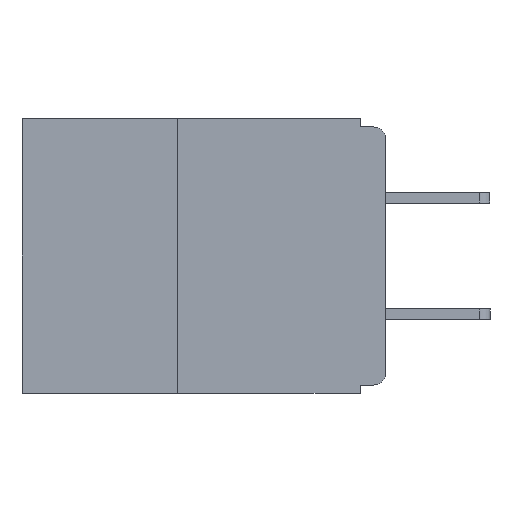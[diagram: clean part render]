
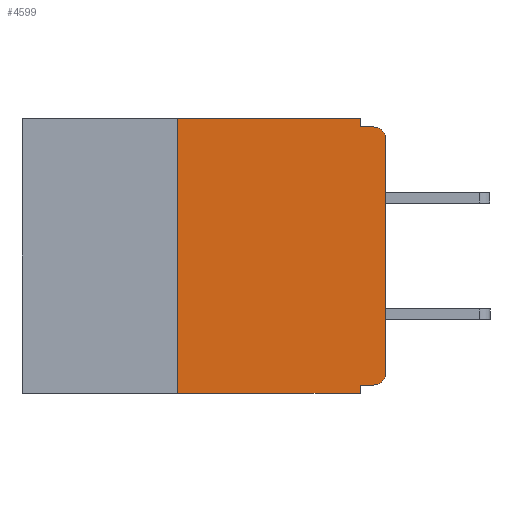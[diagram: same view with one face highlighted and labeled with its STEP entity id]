
A CAD part, left-side view. The second image highlights one B-rep face of the part: STEP entity #4599.
In plain terms, the highlighted planar face has unit normal (-1, 0, 0).
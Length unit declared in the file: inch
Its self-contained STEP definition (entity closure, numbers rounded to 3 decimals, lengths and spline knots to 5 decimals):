
#192 = VERTEX_POINT ( 'NONE', #5050 ) ;
#491 = EDGE_CURVE ( 'NONE', #192, #1452, #2452, .T. ) ;
#806 = CARTESIAN_POINT ( 'NONE',  ( 0., 0., -0.025 ) ) ;
#957 = DIRECTION ( 'NONE',  ( 0., 0., -1. ) ) ;
#994 = VERTEX_POINT ( 'NONE', #12717 ) ;
#1406 = VERTEX_POINT ( 'NONE', #1505 ) ;
#1412 = CARTESIAN_POINT ( 'NONE',  ( 0., 0.437, 0. ) ) ;
#1452 = VERTEX_POINT ( 'NONE', #10037 ) ;
#1505 = CARTESIAN_POINT ( 'NONE',  ( 0., 0.015, -0.32 ) ) ;
#1545 = EDGE_CURVE ( 'NONE', #1880, #10157, #11931, .T. ) ;
#1576 = EDGE_CURVE ( 'NONE', #1725, #10157, #11882, .T. ) ;
#1625 = EDGE_CURVE ( 'NONE', #1725, #192, #11716, .T. ) ;
#1690 = EDGE_CURVE ( 'NONE', #1452, #994, #11460, .T. ) ;
#1725 = VERTEX_POINT ( 'NONE', #12535 ) ;
#1880 = VERTEX_POINT ( 'NONE', #5722 ) ;
#2166 = FACE_OUTER_BOUND ( 'NONE', #4834, .T. ) ;
#2429 = VECTOR ( 'NONE', #12900, 39.37008 ) ;
#2452 = LINE ( 'NONE', #1412, #2429 ) ;
#2476 = DIRECTION ( 'NONE',  ( 0., -1., 0. ) ) ;
#2565 = CARTESIAN_POINT ( 'NONE',  ( 0., 0., -0.01 ) ) ;
#2672 = LINE ( 'NONE', #12463, #2685 ) ;
#2685 = VECTOR ( 'NONE', #12782, 39.37008 ) ;
#3017 = CARTESIAN_POINT ( 'NONE',  ( 0., 0., -0.305 ) ) ;
#3149 = ORIENTED_EDGE ( 'NONE', *, *, #4447, .T. ) ;
#3379 = ORIENTED_EDGE ( 'NONE', *, *, #4062, .T. ) ;
#3480 = VECTOR ( 'NONE', #2476, 39.37008 ) ;
#3514 = LINE ( 'NONE', #2565, #3480 ) ;
#3877 = DIRECTION ( 'NONE',  ( 0., 0., -1. ) ) ;
#3933 = ORIENTED_EDGE ( 'NONE', *, *, #4244, .F. ) ;
#3940 = EDGE_CURVE ( 'NONE', #1406, #6555, #4817, .T. ) ;
#3943 = VECTOR ( 'NONE', #5995, 39.37008 ) ;
#3979 = LINE ( 'NONE', #6008, #3943 ) ;
#4062 = EDGE_CURVE ( 'NONE', #4262, #10025, #4251, .T. ) ;
#4150 = EDGE_CURVE ( 'NONE', #1406, #1880, #3979, .T. ) ;
#4244 = EDGE_CURVE ( 'NONE', #994, #10025, #3514, .T. ) ;
#4251 = CIRCLE ( 'NONE', #8139, 0.015 ) ;
#4262 = VERTEX_POINT ( 'NONE', #806 ) ;
#4311 = CARTESIAN_POINT ( 'NONE',  ( 0., 0.031, -0.33 ) ) ;
#4374 = CARTESIAN_POINT ( 'NONE',  ( 0., 0.031, -0.33 ) ) ;
#4447 = EDGE_CURVE ( 'NONE', #6555, #4262, #2672, .T. ) ;
#4497 = ORIENTED_EDGE ( 'NONE', *, *, #1690, .F. ) ;
#4599 = ADVANCED_FACE ( 'NONE', ( #2166 ), #10645, .F. ) ;
#4693 = ORIENTED_EDGE ( 'NONE', *, *, #491, .F. ) ;
#4733 = AXIS2_PLACEMENT_3D ( 'NONE', #10711, #11013, #10520 ) ;
#4817 = CIRCLE ( 'NONE', #7723, 0.015 ) ;
#4834 = EDGE_LOOP ( 'NONE', ( #3149, #3379, #3933, #4497, #4693, #4862, #5361, #5424, #5799, #7075 ) ) ;
#4862 = ORIENTED_EDGE ( 'NONE', *, *, #1625, .F. ) ;
#5050 = CARTESIAN_POINT ( 'NONE',  ( 0., 0.25, 0. ) ) ;
#5361 = ORIENTED_EDGE ( 'NONE', *, *, #1576, .T. ) ;
#5424 = ORIENTED_EDGE ( 'NONE', *, *, #1545, .F. ) ;
#5722 = CARTESIAN_POINT ( 'NONE',  ( 0., 0.031, -0.32 ) ) ;
#5799 = ORIENTED_EDGE ( 'NONE', *, *, #4150, .F. ) ;
#5995 = DIRECTION ( 'NONE',  ( 0., 1., 0. ) ) ;
#6008 = CARTESIAN_POINT ( 'NONE',  ( 0., 0., -0.32 ) ) ;
#6218 = CARTESIAN_POINT ( 'NONE',  ( 0., 0.015, -0.01 ) ) ;
#6555 = VERTEX_POINT ( 'NONE', #3017 ) ;
#6967 = CARTESIAN_POINT ( 'NONE',  ( 0., 0.25, -0.33 ) ) ;
#7075 = ORIENTED_EDGE ( 'NONE', *, *, #3940, .T. ) ;
#7100 = DIRECTION ( 'NONE',  ( 0., 0., 1. ) ) ;
#7723 = AXIS2_PLACEMENT_3D ( 'NONE', #12375, #12360, #12175 ) ;
#8139 = AXIS2_PLACEMENT_3D ( 'NONE', #8275, #8225, #8173 ) ;
#8173 = DIRECTION ( 'NONE',  ( 0., 0., -1. ) ) ;
#8225 = DIRECTION ( 'NONE',  ( -1., 0., 0. ) ) ;
#8275 = CARTESIAN_POINT ( 'NONE',  ( 0., 0.015, -0.025 ) ) ;
#10025 = VERTEX_POINT ( 'NONE', #6218 ) ;
#10037 = CARTESIAN_POINT ( 'NONE',  ( 0., 0.031, 0. ) ) ;
#10157 = VERTEX_POINT ( 'NONE', #4311 ) ;
#10520 = DIRECTION ( 'NONE',  ( 0., 0., -1. ) ) ;
#10645 = PLANE ( 'NONE',  #4733 ) ;
#10711 = CARTESIAN_POINT ( 'NONE',  ( 0., 0.437, 0. ) ) ;
#11013 = DIRECTION ( 'NONE',  ( 1., 0., 0. ) ) ;
#11460 = LINE ( 'NONE', #13231, #11469 ) ;
#11469 = VECTOR ( 'NONE', #957, 39.37008 ) ;
#11642 = VECTOR ( 'NONE', #7100, 39.37008 ) ;
#11716 = LINE ( 'NONE', #6967, #11642 ) ;
#11765 = VECTOR ( 'NONE', #12724, 39.37008 ) ;
#11857 = VECTOR ( 'NONE', #3877, 39.37008 ) ;
#11882 = LINE ( 'NONE', #13230, #11765 ) ;
#11931 = LINE ( 'NONE', #4374, #11857 ) ;
#12175 = DIRECTION ( 'NONE',  ( 0., 0., -1. ) ) ;
#12360 = DIRECTION ( 'NONE',  ( -1., 0., 0. ) ) ;
#12375 = CARTESIAN_POINT ( 'NONE',  ( 0., 0.015, -0.305 ) ) ;
#12463 = CARTESIAN_POINT ( 'NONE',  ( 0., 0., 0. ) ) ;
#12535 = CARTESIAN_POINT ( 'NONE',  ( 0., 0.25, -0.33 ) ) ;
#12717 = CARTESIAN_POINT ( 'NONE',  ( 0., 0.031, -0.01 ) ) ;
#12724 = DIRECTION ( 'NONE',  ( 0., -1., 0. ) ) ;
#12782 = DIRECTION ( 'NONE',  ( 0., 0., 1. ) ) ;
#12900 = DIRECTION ( 'NONE',  ( 0., -1., 0. ) ) ;
#13230 = CARTESIAN_POINT ( 'NONE',  ( 0., 0.437, -0.33 ) ) ;
#13231 = CARTESIAN_POINT ( 'NONE',  ( 0., 0.031, 0. ) ) ;
